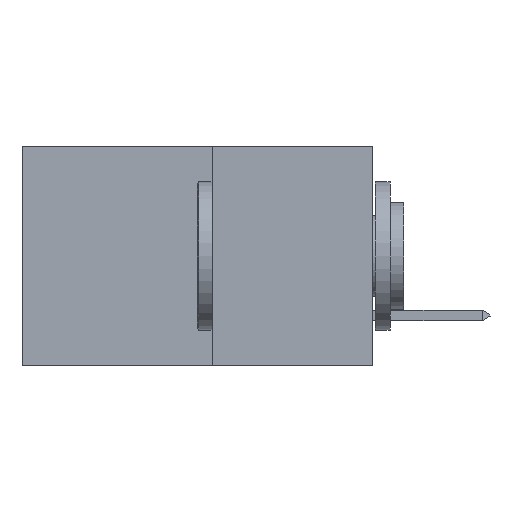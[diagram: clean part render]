
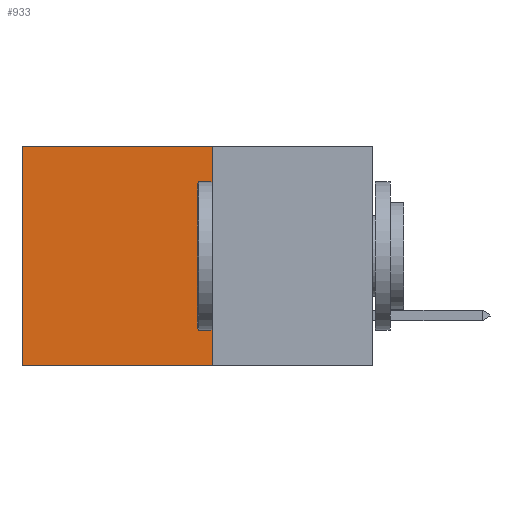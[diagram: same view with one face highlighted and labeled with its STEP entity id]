
A CAD part, left-side view. The second image highlights one B-rep face of the part: STEP entity #933.
In plain terms, the highlighted planar face has unit normal (-1, 0, 0).
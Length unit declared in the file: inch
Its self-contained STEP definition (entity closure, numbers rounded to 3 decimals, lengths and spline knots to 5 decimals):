
#452 = LINE ( 'NONE', #6965, #19867 ) ;
#933 = ADVANCED_FACE ( 'NONE', ( #19013 ), #10141, .F. ) ;
#1250 = CARTESIAN_POINT ( 'NONE',  ( 0.277, 0.27, 0. ) ) ;
#2534 = EDGE_CURVE ( 'NONE', #7076, #14088, #11815, .T. ) ;
#2752 = VERTEX_POINT ( 'NONE', #19278 ) ;
#2952 = LINE ( 'NONE', #11872, #13000 ) ;
#3345 = CARTESIAN_POINT ( 'NONE',  ( 0.277, 0.27, -0.37 ) ) ;
#3890 = DIRECTION ( 'NONE',  ( 0., 0., -1. ) ) ;
#6920 = CARTESIAN_POINT ( 'NONE',  ( 0.277, 0.27, -0.37 ) ) ;
#6944 = VECTOR ( 'NONE', #21278, 39.37008 ) ;
#6965 = CARTESIAN_POINT ( 'NONE',  ( 0.277, 0.27, -0.37 ) ) ;
#7076 = VERTEX_POINT ( 'NONE', #17008 ) ;
#7341 = EDGE_CURVE ( 'NONE', #2752, #12290, #2952, .T. ) ;
#7892 = EDGE_LOOP ( 'NONE', ( #14484, #9228, #12985, #9998 ) ) ;
#8698 = AXIS2_PLACEMENT_3D ( 'NONE', #3345, #23888, #23854 ) ;
#9228 = ORIENTED_EDGE ( 'NONE', *, *, #11992, .F. ) ;
#9816 = EDGE_CURVE ( 'NONE', #7076, #2752, #12236, .T. ) ;
#9998 = ORIENTED_EDGE ( 'NONE', *, *, #9816, .T. ) ;
#10141 = PLANE ( 'NONE',  #8698 ) ;
#11815 = LINE ( 'NONE', #18467, #21754 ) ;
#11872 = CARTESIAN_POINT ( 'NONE',  ( 0.277, 0.59, -0.37 ) ) ;
#11992 = EDGE_CURVE ( 'NONE', #14088, #12290, #452, .T. ) ;
#12236 = LINE ( 'NONE', #1250, #6944 ) ;
#12290 = VERTEX_POINT ( 'NONE', #16007 ) ;
#12985 = ORIENTED_EDGE ( 'NONE', *, *, #2534, .F. ) ;
#13000 = VECTOR ( 'NONE', #3890, 39.37008 ) ;
#14088 = VERTEX_POINT ( 'NONE', #6920 ) ;
#14484 = ORIENTED_EDGE ( 'NONE', *, *, #7341, .T. ) ;
#16007 = CARTESIAN_POINT ( 'NONE',  ( 0.277, 0.59, -0.37 ) ) ;
#16876 = DIRECTION ( 'NONE',  ( 0., 1., 0. ) ) ;
#17008 = CARTESIAN_POINT ( 'NONE',  ( 0.277, 0.27, 0. ) ) ;
#18467 = CARTESIAN_POINT ( 'NONE',  ( 0.277, 0.27, -0.37 ) ) ;
#19013 = FACE_OUTER_BOUND ( 'NONE', #7892, .T. ) ;
#19278 = CARTESIAN_POINT ( 'NONE',  ( 0.277, 0.59, 0. ) ) ;
#19867 = VECTOR ( 'NONE', #16876, 39.37008 ) ;
#21278 = DIRECTION ( 'NONE',  ( 0., 1., 0. ) ) ;
#21282 = DIRECTION ( 'NONE',  ( 0., 0., -1. ) ) ;
#21754 = VECTOR ( 'NONE', #21282, 39.37008 ) ;
#23854 = DIRECTION ( 'NONE',  ( 0., 0., -1. ) ) ;
#23888 = DIRECTION ( 'NONE',  ( 1., 0., 0. ) ) ;
